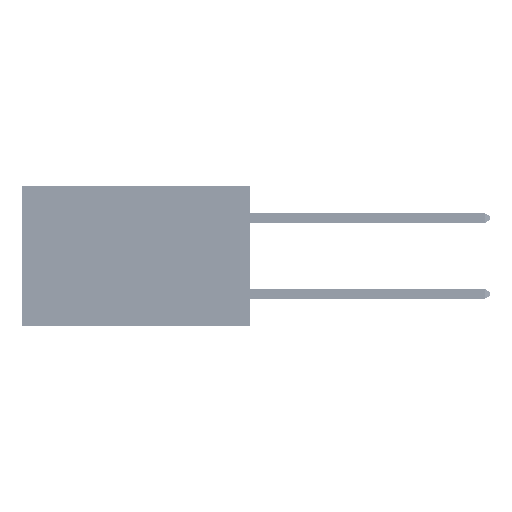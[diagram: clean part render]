
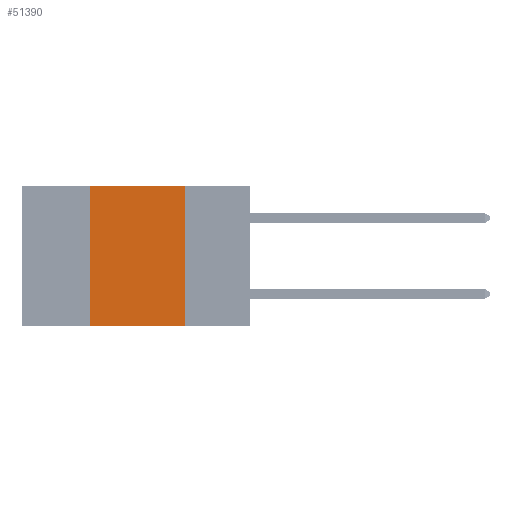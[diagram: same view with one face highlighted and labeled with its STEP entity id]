
A CAD part, left-side view. The second image highlights one B-rep face of the part: STEP entity #51390.
In plain terms, the highlighted planar face has unit normal (-1, 0, 0).
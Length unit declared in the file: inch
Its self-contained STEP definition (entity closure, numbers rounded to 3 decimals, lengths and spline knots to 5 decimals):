
#526 = EDGE_CURVE ( 'NONE', #43580, #7962, #10522, .T. ) ;
#2088 = CARTESIAN_POINT ( 'NONE',  ( 0., 0.17, -0.37 ) ) ;
#3288 = CARTESIAN_POINT ( 'NONE',  ( 0., 0.42, 0. ) ) ;
#3927 = FACE_OUTER_BOUND ( 'NONE', #6731, .T. ) ;
#4194 = DIRECTION ( 'NONE',  ( 0., 0., -1. ) ) ;
#6731 = EDGE_LOOP ( 'NONE', ( #14902, #42787, #47922, #49117 ) ) ;
#7962 = VERTEX_POINT ( 'NONE', #2088 ) ;
#10522 = LINE ( 'NONE', #42093, #22917 ) ;
#11137 = CARTESIAN_POINT ( 'NONE',  ( 0., 0.17, 0. ) ) ;
#11210 = CARTESIAN_POINT ( 'NONE',  ( 0., 0.17, 0. ) ) ;
#11564 = VERTEX_POINT ( 'NONE', #3288 ) ;
#12165 = PLANE ( 'NONE',  #41354 ) ;
#14902 = ORIENTED_EDGE ( 'NONE', *, *, #18770, .F. ) ;
#15743 = CARTESIAN_POINT ( 'NONE',  ( 0., 0.6, 0. ) ) ;
#17798 = LINE ( 'NONE', #42203, #46153 ) ;
#18770 = EDGE_CURVE ( 'NONE', #29855, #7962, #30765, .T. ) ;
#22917 = VECTOR ( 'NONE', #26193, 39.37008 ) ;
#23154 = CARTESIAN_POINT ( 'NONE',  ( 0., 0.42, 0. ) ) ;
#26193 = DIRECTION ( 'NONE',  ( 0., -1., 0. ) ) ;
#26297 = DIRECTION ( 'NONE',  ( 0., -1., 0. ) ) ;
#27315 = DIRECTION ( 'NONE',  ( 0., 0., -1. ) ) ;
#29855 = VERTEX_POINT ( 'NONE', #11210 ) ;
#30107 = EDGE_CURVE ( 'NONE', #11564, #29855, #17798, .T. ) ;
#30666 = VECTOR ( 'NONE', #47558, 39.37008 ) ;
#30765 = LINE ( 'NONE', #11137, #49348 ) ;
#32313 = DIRECTION ( 'NONE',  ( 1., 0., 0. ) ) ;
#32509 = CARTESIAN_POINT ( 'NONE',  ( 0., 0.42, -0.37 ) ) ;
#40330 = EDGE_CURVE ( 'NONE', #43580, #11564, #40354, .T. ) ;
#40354 = LINE ( 'NONE', #23154, #30666 ) ;
#41354 = AXIS2_PLACEMENT_3D ( 'NONE', #15743, #32313, #4194 ) ;
#42093 = CARTESIAN_POINT ( 'NONE',  ( 0., 0.6, -0.37 ) ) ;
#42203 = CARTESIAN_POINT ( 'NONE',  ( 0., 0.6, 0. ) ) ;
#42787 = ORIENTED_EDGE ( 'NONE', *, *, #30107, .F. ) ;
#43580 = VERTEX_POINT ( 'NONE', #32509 ) ;
#46153 = VECTOR ( 'NONE', #26297, 39.37008 ) ;
#47558 = DIRECTION ( 'NONE',  ( 0., 0., 1. ) ) ;
#47922 = ORIENTED_EDGE ( 'NONE', *, *, #40330, .F. ) ;
#49117 = ORIENTED_EDGE ( 'NONE', *, *, #526, .T. ) ;
#49348 = VECTOR ( 'NONE', #27315, 39.37008 ) ;
#51390 = ADVANCED_FACE ( 'NONE', ( #3927 ), #12165, .F. ) ;
